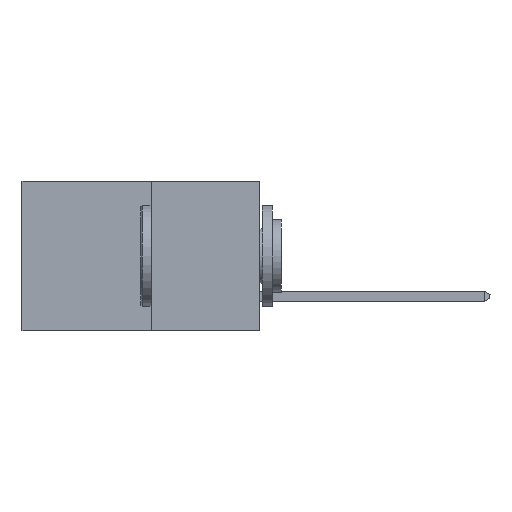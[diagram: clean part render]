
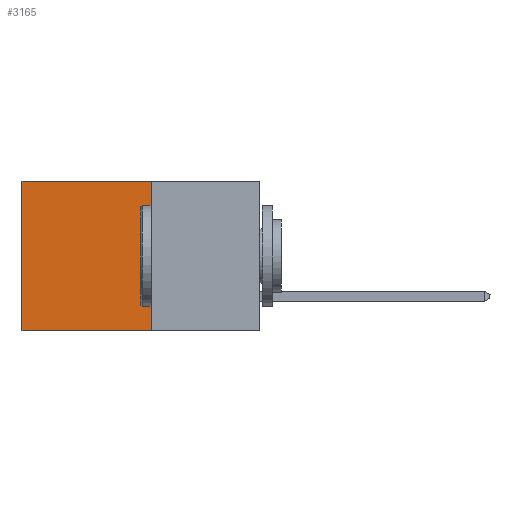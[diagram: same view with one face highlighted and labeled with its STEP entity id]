
A CAD part, left-side view. The second image highlights one B-rep face of the part: STEP entity #3165.
In plain terms, the highlighted planar face has unit normal (-1, 0, 0).
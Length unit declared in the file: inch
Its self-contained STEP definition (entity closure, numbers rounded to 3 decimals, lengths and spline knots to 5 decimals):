
#266 = VECTOR ( 'NONE', #3410, 39.37008 ) ;
#931 = VECTOR ( 'NONE', #13672, 39.37008 ) ;
#1756 = FACE_OUTER_BOUND ( 'NONE', #5003, .T. ) ;
#1925 = CARTESIAN_POINT ( 'NONE',  ( 0.277, 0.27, -0.37 ) ) ;
#2753 = ORIENTED_EDGE ( 'NONE', *, *, #3288, .T. ) ;
#3165 = ADVANCED_FACE ( 'NONE', ( #1756 ), #10329, .F. ) ;
#3288 = EDGE_CURVE ( 'NONE', #4557, #3670, #13251, .T. ) ;
#3410 = DIRECTION ( 'NONE',  ( 0., 1., 0. ) ) ;
#3645 = CARTESIAN_POINT ( 'NONE',  ( 0.277, 0.27, 0. ) ) ;
#3670 = VERTEX_POINT ( 'NONE', #10022 ) ;
#3868 = VECTOR ( 'NONE', #4623, 39.37008 ) ;
#4557 = VERTEX_POINT ( 'NONE', #5350 ) ;
#4623 = DIRECTION ( 'NONE',  ( 0., 0., -1. ) ) ;
#4640 = CARTESIAN_POINT ( 'NONE',  ( 0.277, 0.59, -0.37 ) ) ;
#5003 = EDGE_LOOP ( 'NONE', ( #2753, #5978, #12923, #5426 ) ) ;
#5036 = VECTOR ( 'NONE', #5497, 39.37008 ) ;
#5350 = CARTESIAN_POINT ( 'NONE',  ( 0.277, 0.59, 0. ) ) ;
#5426 = ORIENTED_EDGE ( 'NONE', *, *, #7106, .T. ) ;
#5497 = DIRECTION ( 'NONE',  ( 0., 1., 0. ) ) ;
#5978 = ORIENTED_EDGE ( 'NONE', *, *, #12398, .F. ) ;
#6028 = VERTEX_POINT ( 'NONE', #15328 ) ;
#6171 = EDGE_CURVE ( 'NONE', #6028, #8076, #7815, .T. ) ;
#7106 = EDGE_CURVE ( 'NONE', #6028, #4557, #8855, .T. ) ;
#7815 = LINE ( 'NONE', #13586, #931 ) ;
#8076 = VERTEX_POINT ( 'NONE', #1925 ) ;
#8181 = LINE ( 'NONE', #12457, #5036 ) ;
#8855 = LINE ( 'NONE', #3645, #266 ) ;
#9629 = DIRECTION ( 'NONE',  ( 0., 0., -1. ) ) ;
#9656 = DIRECTION ( 'NONE',  ( 1., 0., 0. ) ) ;
#9796 = CARTESIAN_POINT ( 'NONE',  ( 0.277, 0.27, -0.37 ) ) ;
#10022 = CARTESIAN_POINT ( 'NONE',  ( 0.277, 0.59, -0.37 ) ) ;
#10329 = PLANE ( 'NONE',  #15141 ) ;
#12398 = EDGE_CURVE ( 'NONE', #8076, #3670, #8181, .T. ) ;
#12457 = CARTESIAN_POINT ( 'NONE',  ( 0.277, 0.27, -0.37 ) ) ;
#12923 = ORIENTED_EDGE ( 'NONE', *, *, #6171, .F. ) ;
#13251 = LINE ( 'NONE', #4640, #3868 ) ;
#13586 = CARTESIAN_POINT ( 'NONE',  ( 0.277, 0.27, -0.37 ) ) ;
#13672 = DIRECTION ( 'NONE',  ( 0., 0., -1. ) ) ;
#15141 = AXIS2_PLACEMENT_3D ( 'NONE', #9796, #9656, #9629 ) ;
#15328 = CARTESIAN_POINT ( 'NONE',  ( 0.277, 0.27, 0. ) ) ;
